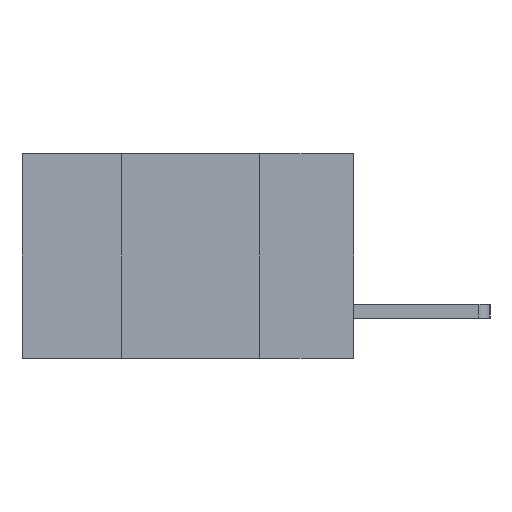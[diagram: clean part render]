
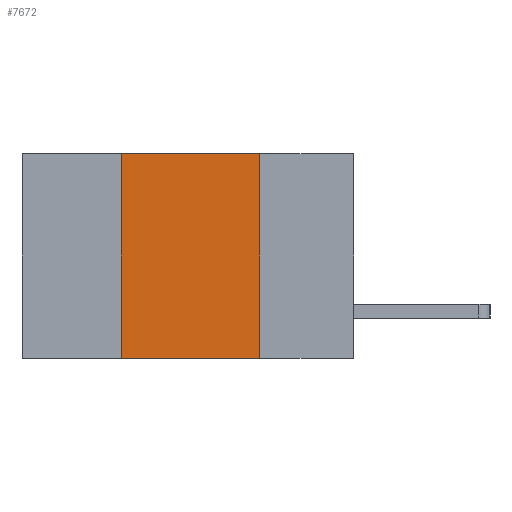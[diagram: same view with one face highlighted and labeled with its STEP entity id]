
A CAD part, left-side view. The second image highlights one B-rep face of the part: STEP entity #7672.
In plain terms, the highlighted planar face has unit normal (-1, 0, 0).
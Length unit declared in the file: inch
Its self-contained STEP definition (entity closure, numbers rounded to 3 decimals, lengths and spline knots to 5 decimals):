
#169 = ORIENTED_EDGE ( 'NONE', *, *, #3353, .F. ) ;
#391 = VERTEX_POINT ( 'NONE', #7332 ) ;
#419 = DIRECTION ( 'NONE',  ( 0., -1., 0. ) ) ;
#446 = VECTOR ( 'NONE', #7678, 39.37008 ) ;
#467 = CARTESIAN_POINT ( 'NONE',  ( 0., 0.6, 0. ) ) ;
#564 = CARTESIAN_POINT ( 'NONE',  ( 0., 0.6, -0.37 ) ) ;
#617 = CARTESIAN_POINT ( 'NONE',  ( 0., 0.6, 0. ) ) ;
#641 = VERTEX_POINT ( 'NONE', #5032 ) ;
#1479 = EDGE_LOOP ( 'NONE', ( #169, #1820, #3684, #6766 ) ) ;
#1820 = ORIENTED_EDGE ( 'NONE', *, *, #7824, .F. ) ;
#2089 = DIRECTION ( 'NONE',  ( 1., 0., 0. ) ) ;
#2193 = LINE ( 'NONE', #564, #9276 ) ;
#2243 = LINE ( 'NONE', #617, #3071 ) ;
#2656 = VERTEX_POINT ( 'NONE', #8802 ) ;
#2793 = CARTESIAN_POINT ( 'NONE',  ( 0., 0.17, -0.37 ) ) ;
#3071 = VECTOR ( 'NONE', #3257, 39.37008 ) ;
#3257 = DIRECTION ( 'NONE',  ( 0., -1., 0. ) ) ;
#3353 = EDGE_CURVE ( 'NONE', #2656, #8828, #8210, .T. ) ;
#3684 = ORIENTED_EDGE ( 'NONE', *, *, #6416, .F. ) ;
#4660 = PLANE ( 'NONE',  #10274 ) ;
#5032 = CARTESIAN_POINT ( 'NONE',  ( 0., 0.42, 0. ) ) ;
#5202 = DIRECTION ( 'NONE',  ( 0., 0., 1. ) ) ;
#6416 = EDGE_CURVE ( 'NONE', #391, #641, #6821, .T. ) ;
#6766 = ORIENTED_EDGE ( 'NONE', *, *, #10323, .T. ) ;
#6775 = CARTESIAN_POINT ( 'NONE',  ( 0., 0.42, 0. ) ) ;
#6821 = LINE ( 'NONE', #6775, #9925 ) ;
#6940 = DIRECTION ( 'NONE',  ( 0., 0., -1. ) ) ;
#7332 = CARTESIAN_POINT ( 'NONE',  ( 0., 0.42, -0.37 ) ) ;
#7672 = ADVANCED_FACE ( 'NONE', ( #8678 ), #4660, .F. ) ;
#7678 = DIRECTION ( 'NONE',  ( 0., 0., -1. ) ) ;
#7824 = EDGE_CURVE ( 'NONE', #641, #2656, #2243, .T. ) ;
#8210 = LINE ( 'NONE', #8431, #446 ) ;
#8431 = CARTESIAN_POINT ( 'NONE',  ( 0., 0.17, 0. ) ) ;
#8678 = FACE_OUTER_BOUND ( 'NONE', #1479, .T. ) ;
#8802 = CARTESIAN_POINT ( 'NONE',  ( 0., 0.17, 0. ) ) ;
#8828 = VERTEX_POINT ( 'NONE', #2793 ) ;
#9276 = VECTOR ( 'NONE', #419, 39.37008 ) ;
#9925 = VECTOR ( 'NONE', #5202, 39.37008 ) ;
#10274 = AXIS2_PLACEMENT_3D ( 'NONE', #467, #2089, #6940 ) ;
#10323 = EDGE_CURVE ( 'NONE', #391, #8828, #2193, .T. ) ;
